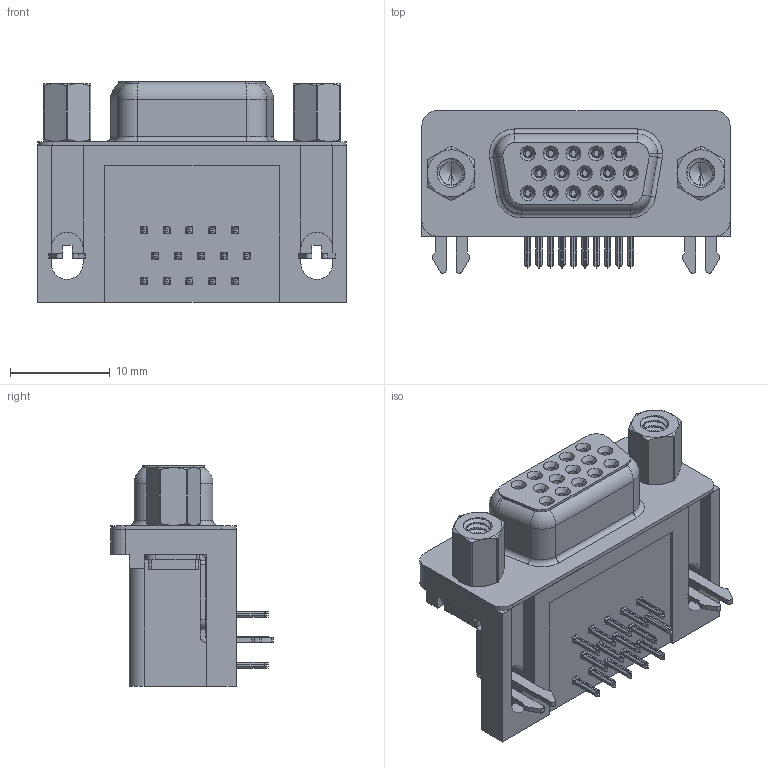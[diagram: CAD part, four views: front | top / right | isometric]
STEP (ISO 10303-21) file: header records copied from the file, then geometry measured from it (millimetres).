
FILE_DESCRIPTION (( 'STEP AP203' ), '1' );
FILE_NAME ('634-015-374-033.STEP', '2018-08-17T23:03:03', ( '' ), ( '' ), 'SwSTEP 2.0', 'SolidWorks 2016', '' );
FILE_SCHEMA (( 'CONFIG_CONTROL_DESIGN' ));
Length unit declared in the file: millimetre
Products named in the file (10): 4-40 Hex Standoff; Contact Bottom; 634-015-374-033; Contact Middle; Contact Top; 2 Prong Board Lock; Contact Middle_Recessed; 634 Housing; 4-40 Threaded Rivet; 634 Shell
Assembly tree (23 placements, depth 2):
  634-015-374-033
    634 Housing
    634 Shell
    Contact Bottom  x5
    Contact Middle  x4
    Contact Top  x5
    2 Prong Board Lock  x2
    Contact Middle_Recessed
    4-40 Threaded Rivet  x2
    4-40 Hex Standoff  x2
Bounding box: 30.89 x 16.25 x 22.1 mm (x, y, z)
Volume: 4754.4 mm3; surface area: 6955.9 mm2
Topology: 23 solids, 23 shells, 2581 faces, 6814 edges, 4296 vertices
Faces by surface type: plane 1120, cylinder 671, bspline 538, cone 214, torus 38
Entity records: 42075 total; most frequent: CARTESIAN_POINT 16841, ORIENTED_EDGE 5342, DIRECTION 4356, EDGE_CURVE 2671, VERTEX_POINT 1700, LINE 1552, VECTOR 1552, AXIS2_PLACEMENT_3D 1402
